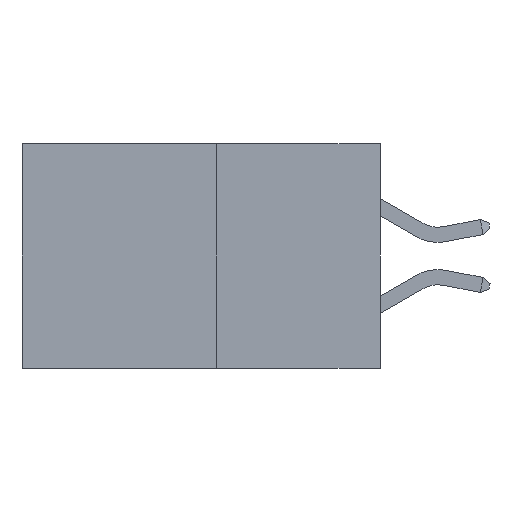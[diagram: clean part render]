
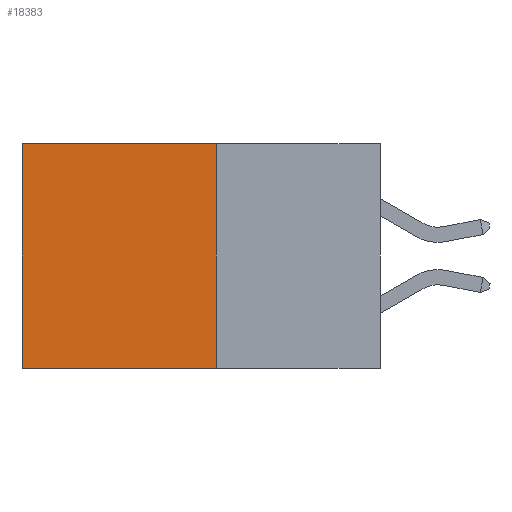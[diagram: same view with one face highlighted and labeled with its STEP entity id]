
A CAD part, left-side view. The second image highlights one B-rep face of the part: STEP entity #18383.
In plain terms, the highlighted planar face has unit normal (-1, 0, 0).
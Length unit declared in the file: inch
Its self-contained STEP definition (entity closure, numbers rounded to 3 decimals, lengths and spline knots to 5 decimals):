
#218 = VERTEX_POINT ( 'NONE', #11314 ) ;
#911 = DIRECTION ( 'NONE',  ( 0., 0., -1. ) ) ;
#1194 = EDGE_CURVE ( 'NONE', #218, #16406, #20676, .T. ) ;
#1374 = AXIS2_PLACEMENT_3D ( 'NONE', #16056, #12820, #3030 ) ;
#1502 = EDGE_CURVE ( 'NONE', #16406, #2029, #6904, .T. ) ;
#1938 = FACE_OUTER_BOUND ( 'NONE', #12924, .T. ) ;
#1971 = CARTESIAN_POINT ( 'NONE',  ( 0.277, 0.27, -0.37 ) ) ;
#2029 = VERTEX_POINT ( 'NONE', #17314 ) ;
#3030 = DIRECTION ( 'NONE',  ( 0., 0., -1. ) ) ;
#3356 = VECTOR ( 'NONE', #6533, 39.37008 ) ;
#4383 = CARTESIAN_POINT ( 'NONE',  ( 0.277, 0.27, -0.37 ) ) ;
#6533 = DIRECTION ( 'NONE',  ( 0., 1., 0. ) ) ;
#6868 = CARTESIAN_POINT ( 'NONE',  ( 0.277, 0.59, 0. ) ) ;
#6904 = LINE ( 'NONE', #1971, #14639 ) ;
#9434 = PLANE ( 'NONE',  #1374 ) ;
#10653 = CARTESIAN_POINT ( 'NONE',  ( 0.277, 0.59, -0.37 ) ) ;
#11044 = VECTOR ( 'NONE', #12280, 39.37008 ) ;
#11289 = VERTEX_POINT ( 'NONE', #6868 ) ;
#11314 = CARTESIAN_POINT ( 'NONE',  ( 0.277, 0.27, 0. ) ) ;
#12068 = VECTOR ( 'NONE', #911, 39.37008 ) ;
#12280 = DIRECTION ( 'NONE',  ( 0., 0., -1. ) ) ;
#12794 = EDGE_CURVE ( 'NONE', #11289, #2029, #19186, .T. ) ;
#12820 = DIRECTION ( 'NONE',  ( 1., 0., 0. ) ) ;
#12924 = EDGE_LOOP ( 'NONE', ( #18684, #18877, #16456, #13237 ) ) ;
#13140 = EDGE_CURVE ( 'NONE', #218, #11289, #20660, .T. ) ;
#13237 = ORIENTED_EDGE ( 'NONE', *, *, #13140, .T. ) ;
#14639 = VECTOR ( 'NONE', #16243, 39.37008 ) ;
#16056 = CARTESIAN_POINT ( 'NONE',  ( 0.277, 0.27, -0.37 ) ) ;
#16243 = DIRECTION ( 'NONE',  ( 0., 1., 0. ) ) ;
#16406 = VERTEX_POINT ( 'NONE', #4383 ) ;
#16456 = ORIENTED_EDGE ( 'NONE', *, *, #1194, .F. ) ;
#17314 = CARTESIAN_POINT ( 'NONE',  ( 0.277, 0.59, -0.37 ) ) ;
#17979 = CARTESIAN_POINT ( 'NONE',  ( 0.277, 0.27, 0. ) ) ;
#18296 = CARTESIAN_POINT ( 'NONE',  ( 0.277, 0.27, -0.37 ) ) ;
#18383 = ADVANCED_FACE ( 'NONE', ( #1938 ), #9434, .F. ) ;
#18684 = ORIENTED_EDGE ( 'NONE', *, *, #12794, .T. ) ;
#18877 = ORIENTED_EDGE ( 'NONE', *, *, #1502, .F. ) ;
#19186 = LINE ( 'NONE', #10653, #11044 ) ;
#20660 = LINE ( 'NONE', #17979, #3356 ) ;
#20676 = LINE ( 'NONE', #18296, #12068 ) ;
